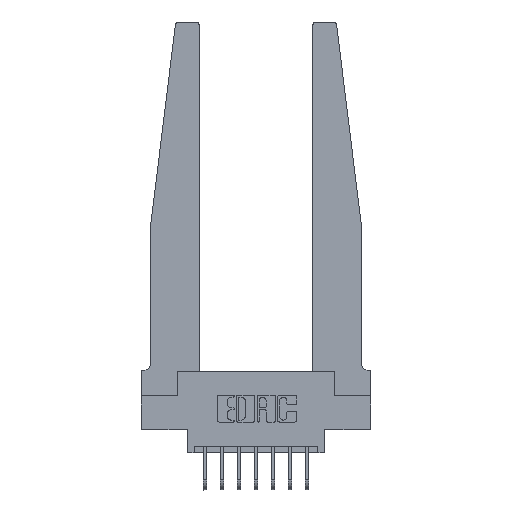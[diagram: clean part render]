
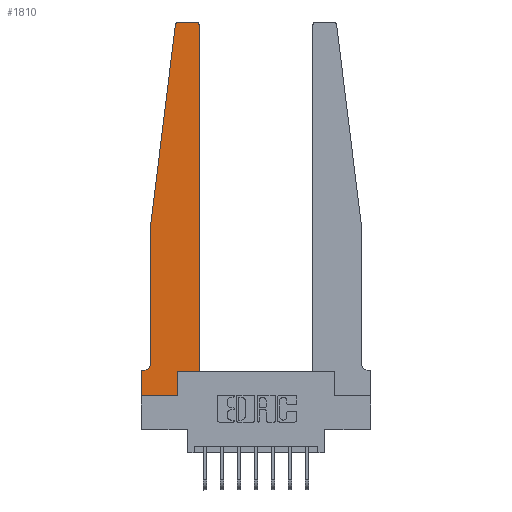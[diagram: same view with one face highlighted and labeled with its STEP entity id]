
A CAD part, top view. The second image highlights one B-rep face of the part: STEP entity #1810.
In plain terms, the highlighted planar face has unit normal (0, 0, 1).
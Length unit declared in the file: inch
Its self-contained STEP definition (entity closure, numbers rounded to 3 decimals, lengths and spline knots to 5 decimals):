
#98 = DIRECTION ( 'NONE',  ( 0., 0., -1. ) ) ;
#113 = ORIENTED_EDGE ( 'NONE', *, *, #11009, .T. ) ;
#153 = VECTOR ( 'NONE', #4208, 39.37008 ) ;
#154 = DIRECTION ( 'NONE',  ( 0., 0., 1. ) ) ;
#614 = AXIS2_PLACEMENT_3D ( 'NONE', #2645, #98, #8703 ) ;
#787 = ORIENTED_EDGE ( 'NONE', *, *, #7663, .T. ) ;
#940 = VECTOR ( 'NONE', #12229, 39.37008 ) ;
#1377 = DIRECTION ( 'NONE',  ( 0., -1., 0. ) ) ;
#1709 = AXIS2_PLACEMENT_3D ( 'NONE', #12167, #154, #13442 ) ;
#1810 = ADVANCED_FACE ( 'NONE', ( #5380 ), #9050, .T. ) ;
#1985 = CARTESIAN_POINT ( 'NONE',  ( 0.395, 2.72, 0.37 ) ) ;
#1998 = VERTEX_POINT ( 'NONE', #13568 ) ;
#2006 = CARTESIAN_POINT ( 'NONE',  ( 0.24675, 2.72367, 0.37 ) ) ;
#2262 = DIRECTION ( 'NONE',  ( -1., 0., 0. ) ) ;
#2332 = ORIENTED_EDGE ( 'NONE', *, *, #15970, .T. ) ;
#2645 = CARTESIAN_POINT ( 'NONE',  ( 0.015, 0.2375, 0.37 ) ) ;
#2714 = VERTEX_POINT ( 'NONE', #8304 ) ;
#3200 = ORIENTED_EDGE ( 'NONE', *, *, #7305, .T. ) ;
#3544 = CARTESIAN_POINT ( 'NONE',  ( 0.2605, 0.18, 0.37 ) ) ;
#3589 = CARTESIAN_POINT ( 'NONE',  ( 0.065, 0.1875, 0.37 ) ) ;
#3657 = VERTEX_POINT ( 'NONE', #15952 ) ;
#3960 = EDGE_CURVE ( 'NONE', #6857, #9025, #13886, .T. ) ;
#3969 = CARTESIAN_POINT ( 'NONE',  ( 0.065, 1.25, 0.37 ) ) ;
#4150 = LINE ( 'NONE', #3969, #8807 ) ;
#4208 = DIRECTION ( 'NONE',  ( 1., 0., 0. ) ) ;
#4333 = DIRECTION ( 'NONE',  ( 0., 0., 1. ) ) ;
#4441 = DIRECTION ( 'NONE',  ( -1., 0., 0. ) ) ;
#4598 = CARTESIAN_POINT ( 'NONE',  ( 0.065, 0.2375, 0.37 ) ) ;
#4929 = CARTESIAN_POINT ( 'NONE',  ( 0.065, 1.25, 0.37 ) ) ;
#5141 = VECTOR ( 'NONE', #4441, 39.37008 ) ;
#5378 = CARTESIAN_POINT ( 'NONE',  ( 0.425, 0.18, 0.37 ) ) ;
#5380 = FACE_OUTER_BOUND ( 'NONE', #13702, .T. ) ;
#5575 = CARTESIAN_POINT ( 'NONE',  ( 0.425, 0.18, 0.37 ) ) ;
#5747 = ORIENTED_EDGE ( 'NONE', *, *, #8425, .T. ) ;
#6096 = LINE ( 'NONE', #8426, #940 ) ;
#6165 = VERTEX_POINT ( 'NONE', #4598 ) ;
#6592 = LINE ( 'NONE', #3589, #13617 ) ;
#6624 = EDGE_CURVE ( 'NONE', #3657, #6165, #4150, .T. ) ;
#6857 = VERTEX_POINT ( 'NONE', #5575 ) ;
#6938 = ORIENTED_EDGE ( 'NONE', *, *, #14209, .T. ) ;
#7036 = VERTEX_POINT ( 'NONE', #9070 ) ;
#7161 = CARTESIAN_POINT ( 'NONE',  ( 0., 0., 0.37 ) ) ;
#7305 = EDGE_CURVE ( 'NONE', #7036, #7546, #6096, .T. ) ;
#7414 = EDGE_CURVE ( 'NONE', #7546, #6857, #15787, .T. ) ;
#7546 = VERTEX_POINT ( 'NONE', #3544 ) ;
#7616 = LINE ( 'NONE', #7161, #11214 ) ;
#7663 = EDGE_CURVE ( 'NONE', #13850, #7036, #7616, .T. ) ;
#7802 = DIRECTION ( 'NONE',  ( 0., 0., 1. ) ) ;
#7910 = EDGE_CURVE ( 'NONE', #1998, #13850, #13363, .T. ) ;
#8074 = LINE ( 'NONE', #14293, #5141 ) ;
#8304 = CARTESIAN_POINT ( 'NONE',  ( 0.395, 2.75, 0.37 ) ) ;
#8425 = EDGE_CURVE ( 'NONE', #11064, #12082, #11342, .T. ) ;
#8426 = CARTESIAN_POINT ( 'NONE',  ( 0.2605, 0.18, 0.37 ) ) ;
#8703 = DIRECTION ( 'NONE',  ( -1., 0., 0. ) ) ;
#8727 = CARTESIAN_POINT ( 'NONE',  ( 0., 0., 0.37 ) ) ;
#8807 = VECTOR ( 'NONE', #1377, 39.37008 ) ;
#8994 = ORIENTED_EDGE ( 'NONE', *, *, #7910, .T. ) ;
#9025 = VERTEX_POINT ( 'NONE', #13696 ) ;
#9050 = PLANE ( 'NONE',  #13635 ) ;
#9070 = CARTESIAN_POINT ( 'NONE',  ( 0.2605, 0., 0.37 ) ) ;
#9661 = DIRECTION ( 'NONE',  ( 1., 0., 0. ) ) ;
#10375 = VECTOR ( 'NONE', #11888, 39.37008 ) ;
#10472 = DIRECTION ( 'NONE',  ( 1., 0., 0. ) ) ;
#10652 = LINE ( 'NONE', #4929, #13963 ) ;
#10948 = CARTESIAN_POINT ( 'NONE',  ( 0.27653, 2.75, 0.37 ) ) ;
#10986 = DIRECTION ( 'NONE',  ( -0.122, -0.992, 0. ) ) ;
#11009 = EDGE_CURVE ( 'NONE', #12226, #1998, #6592, .T. ) ;
#11017 = AXIS2_PLACEMENT_3D ( 'NONE', #1985, #4333, #10472 ) ;
#11064 = VERTEX_POINT ( 'NONE', #10948 ) ;
#11214 = VECTOR ( 'NONE', #9661, 39.37008 ) ;
#11342 = CIRCLE ( 'NONE', #1709, 0.03 ) ;
#11374 = CARTESIAN_POINT ( 'NONE',  ( 0., 0., 0.37 ) ) ;
#11424 = DIRECTION ( 'NONE',  ( 1., 0., 0. ) ) ;
#11562 = CIRCLE ( 'NONE', #614, 0.05 ) ;
#11765 = EDGE_CURVE ( 'NONE', #12082, #3657, #10652, .T. ) ;
#11888 = DIRECTION ( 'NONE',  ( 0., 1., 0. ) ) ;
#12082 = VERTEX_POINT ( 'NONE', #2006 ) ;
#12167 = CARTESIAN_POINT ( 'NONE',  ( 0.27653, 2.72, 0.37 ) ) ;
#12226 = VERTEX_POINT ( 'NONE', #14728 ) ;
#12229 = DIRECTION ( 'NONE',  ( 0., 1., 0. ) ) ;
#12266 = ORIENTED_EDGE ( 'NONE', *, *, #11765, .T. ) ;
#12558 = VECTOR ( 'NONE', #13061, 39.37008 ) ;
#13061 = DIRECTION ( 'NONE',  ( 0., -1., 0. ) ) ;
#13160 = ORIENTED_EDGE ( 'NONE', *, *, #3960, .T. ) ;
#13269 = CARTESIAN_POINT ( 'NONE',  ( 0.425, 0.18, 0.37 ) ) ;
#13354 = CIRCLE ( 'NONE', #11017, 0.03 ) ;
#13363 = LINE ( 'NONE', #11374, #12558 ) ;
#13442 = DIRECTION ( 'NONE',  ( 1., 0., 0. ) ) ;
#13568 = CARTESIAN_POINT ( 'NONE',  ( 0., 0.1875, 0.37 ) ) ;
#13617 = VECTOR ( 'NONE', #2262, 39.37008 ) ;
#13635 = AXIS2_PLACEMENT_3D ( 'NONE', #13904, #7802, #11424 ) ;
#13696 = CARTESIAN_POINT ( 'NONE',  ( 0.425, 2.72, 0.37 ) ) ;
#13702 = EDGE_LOOP ( 'NONE', ( #6938, #5747, #12266, #15324, #2332, #113, #8994, #787, #3200, #13779, #13160, #15053 ) ) ;
#13779 = ORIENTED_EDGE ( 'NONE', *, *, #7414, .T. ) ;
#13850 = VERTEX_POINT ( 'NONE', #8727 ) ;
#13886 = LINE ( 'NONE', #13269, #10375 ) ;
#13904 = CARTESIAN_POINT ( 'NONE',  ( 0., 0.1875, 0.37 ) ) ;
#13963 = VECTOR ( 'NONE', #10986, 39.37008 ) ;
#14181 = EDGE_CURVE ( 'NONE', #9025, #2714, #13354, .T. ) ;
#14209 = EDGE_CURVE ( 'NONE', #2714, #11064, #8074, .T. ) ;
#14293 = CARTESIAN_POINT ( 'NONE',  ( 0.25, 2.75, 0.37 ) ) ;
#14728 = CARTESIAN_POINT ( 'NONE',  ( 0.015, 0.1875, 0.37 ) ) ;
#15053 = ORIENTED_EDGE ( 'NONE', *, *, #14181, .T. ) ;
#15324 = ORIENTED_EDGE ( 'NONE', *, *, #6624, .T. ) ;
#15787 = LINE ( 'NONE', #5378, #153 ) ;
#15952 = CARTESIAN_POINT ( 'NONE',  ( 0.065, 1.25, 0.37 ) ) ;
#15970 = EDGE_CURVE ( 'NONE', #6165, #12226, #11562, .T. ) ;
